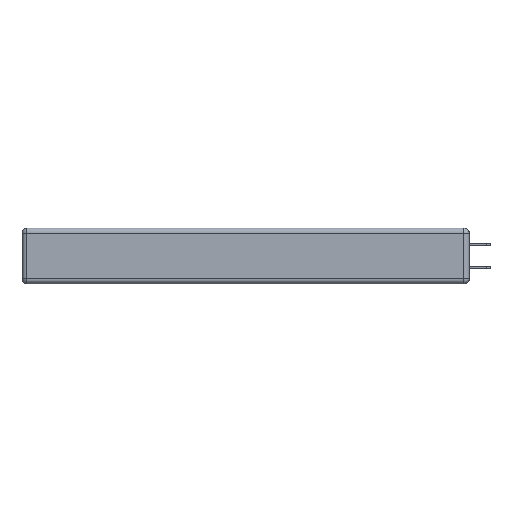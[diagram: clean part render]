
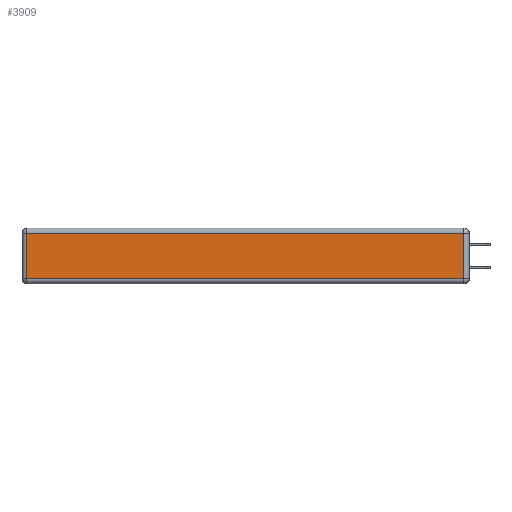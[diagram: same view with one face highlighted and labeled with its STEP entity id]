
A CAD part, left-side view. The second image highlights one B-rep face of the part: STEP entity #3909.
In plain terms, the highlighted planar face has unit normal (-1, 0, 0).
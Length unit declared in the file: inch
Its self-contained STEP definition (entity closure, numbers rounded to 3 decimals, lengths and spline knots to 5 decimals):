
#423 = LINE ( 'NONE', #3377, #7775 ) ;
#696 = VERTEX_POINT ( 'NONE', #11136 ) ;
#1205 = EDGE_CURVE ( 'NONE', #9476, #13414, #423, .T. ) ;
#1238 = EDGE_CURVE ( 'NONE', #13583, #9476, #10192, .T. ) ;
#2140 = VECTOR ( 'NONE', #8748, 39.37008 ) ;
#2385 = ORIENTED_EDGE ( 'NONE', *, *, #1205, .T. ) ;
#2771 = ORIENTED_EDGE ( 'NONE', *, *, #1238, .T. ) ;
#3377 = CARTESIAN_POINT ( 'NONE',  ( 0., 0., -0.313 ) ) ;
#3636 = CARTESIAN_POINT ( 'NONE',  ( 0., 2.75, -0.03 ) ) ;
#3909 = ADVANCED_FACE ( 'NONE', ( #9665 ), #10453, .T. ) ;
#4140 = DIRECTION ( 'NONE',  ( 0., 0., 1. ) ) ;
#4509 = CARTESIAN_POINT ( 'NONE',  ( 0., 2.72, -0.313 ) ) ;
#4823 = DIRECTION ( 'NONE',  ( 0., -1., 0. ) ) ;
#4947 = CARTESIAN_POINT ( 'NONE',  ( 0., 2.72, -0.03 ) ) ;
#5418 = DIRECTION ( 'NONE',  ( -1., 0., 0. ) ) ;
#6556 = CARTESIAN_POINT ( 'NONE',  ( 0., 0., -0.343 ) ) ;
#7165 = CARTESIAN_POINT ( 'NONE',  ( 0., 2.72, -0.343 ) ) ;
#7334 = ORIENTED_EDGE ( 'NONE', *, *, #11396, .T. ) ;
#7775 = VECTOR ( 'NONE', #4823, 39.37008 ) ;
#8196 = DIRECTION ( 'NONE',  ( 0., 0., 1. ) ) ;
#8748 = DIRECTION ( 'NONE',  ( 0., 1., 0. ) ) ;
#8878 = EDGE_CURVE ( 'NONE', #696, #13583, #12100, .T. ) ;
#9222 = ORIENTED_EDGE ( 'NONE', *, *, #8878, .T. ) ;
#9476 = VERTEX_POINT ( 'NONE', #4509 ) ;
#9665 = FACE_OUTER_BOUND ( 'NONE', #12699, .T. ) ;
#9693 = CARTESIAN_POINT ( 'NONE',  ( 0., 0.03, -0.313 ) ) ;
#9887 = AXIS2_PLACEMENT_3D ( 'NONE', #6556, #5418, #4140 ) ;
#10192 = LINE ( 'NONE', #7165, #11971 ) ;
#10453 = PLANE ( 'NONE',  #9887 ) ;
#11136 = CARTESIAN_POINT ( 'NONE',  ( 0., 0.03, -0.03 ) ) ;
#11396 = EDGE_CURVE ( 'NONE', #13414, #696, #12618, .T. ) ;
#11971 = VECTOR ( 'NONE', #13479, 39.37008 ) ;
#12100 = LINE ( 'NONE', #3636, #2140 ) ;
#12233 = VECTOR ( 'NONE', #8196, 39.37008 ) ;
#12618 = LINE ( 'NONE', #13246, #12233 ) ;
#12699 = EDGE_LOOP ( 'NONE', ( #2385, #7334, #9222, #2771 ) ) ;
#13246 = CARTESIAN_POINT ( 'NONE',  ( 0., 0.03, -0.343 ) ) ;
#13414 = VERTEX_POINT ( 'NONE', #9693 ) ;
#13479 = DIRECTION ( 'NONE',  ( 0., 0., -1. ) ) ;
#13583 = VERTEX_POINT ( 'NONE', #4947 ) ;
